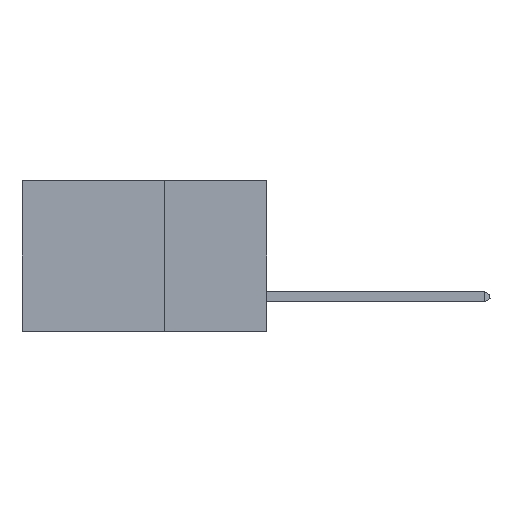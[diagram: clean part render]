
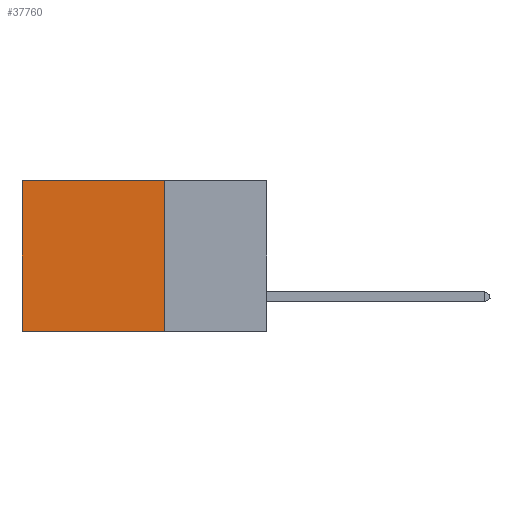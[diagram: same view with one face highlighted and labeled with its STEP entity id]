
A CAD part, left-side view. The second image highlights one B-rep face of the part: STEP entity #37760.
In plain terms, the highlighted planar face has unit normal (-1, 0, 0).
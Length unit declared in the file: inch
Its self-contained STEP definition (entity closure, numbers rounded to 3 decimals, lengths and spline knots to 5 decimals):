
#5475 = VECTOR ( 'NONE', #35200, 39.37008 ) ;
#6870 = VECTOR ( 'NONE', #21908, 39.37008 ) ;
#8122 = CARTESIAN_POINT ( 'NONE',  ( 0.2875, 0.25, 0. ) ) ;
#8589 = FACE_OUTER_BOUND ( 'NONE', #17718, .T. ) ;
#9537 = CARTESIAN_POINT ( 'NONE',  ( 0.2875, 0.25, -0.37 ) ) ;
#10357 = ORIENTED_EDGE ( 'NONE', *, *, #39646, .F. ) ;
#11465 = DIRECTION ( 'NONE',  ( 1., 0., 0. ) ) ;
#13962 = CARTESIAN_POINT ( 'NONE',  ( 0.2875, 0.6, 0. ) ) ;
#14576 = LINE ( 'NONE', #37677, #35954 ) ;
#15510 = EDGE_CURVE ( 'NONE', #18919, #43101, #44362, .T. ) ;
#15926 = CARTESIAN_POINT ( 'NONE',  ( 0.2875, 0.25, 0. ) ) ;
#16821 = LINE ( 'NONE', #13962, #6870 ) ;
#17718 = EDGE_LOOP ( 'NONE', ( #42043, #27806, #10357, #18698 ) ) ;
#17753 = VECTOR ( 'NONE', #43598, 39.37008 ) ;
#18698 = ORIENTED_EDGE ( 'NONE', *, *, #42500, .T. ) ;
#18919 = VERTEX_POINT ( 'NONE', #36435 ) ;
#21020 = EDGE_CURVE ( 'NONE', #38689, #43101, #16821, .T. ) ;
#21908 = DIRECTION ( 'NONE',  ( 0., 0., -1. ) ) ;
#25584 = LINE ( 'NONE', #15926, #5475 ) ;
#27806 = ORIENTED_EDGE ( 'NONE', *, *, #15510, .F. ) ;
#33387 = AXIS2_PLACEMENT_3D ( 'NONE', #8122, #11465, #42192 ) ;
#34142 = PLANE ( 'NONE',  #33387 ) ;
#35200 = DIRECTION ( 'NONE',  ( 0., 0., -1. ) ) ;
#35954 = VECTOR ( 'NONE', #45990, 39.37008 ) ;
#36435 = CARTESIAN_POINT ( 'NONE',  ( 0.2875, 0.25, -0.37 ) ) ;
#37048 = CARTESIAN_POINT ( 'NONE',  ( 0.2875, 0.6, 0. ) ) ;
#37677 = CARTESIAN_POINT ( 'NONE',  ( 0.2875, 0.25, 0. ) ) ;
#37760 = ADVANCED_FACE ( 'NONE', ( #8589 ), #34142, .F. ) ;
#38689 = VERTEX_POINT ( 'NONE', #37048 ) ;
#39646 = EDGE_CURVE ( 'NONE', #40499, #18919, #25584, .T. ) ;
#40436 = CARTESIAN_POINT ( 'NONE',  ( 0.2875, 0.6, -0.37 ) ) ;
#40499 = VERTEX_POINT ( 'NONE', #48067 ) ;
#42043 = ORIENTED_EDGE ( 'NONE', *, *, #21020, .T. ) ;
#42192 = DIRECTION ( 'NONE',  ( 0., 0., -1. ) ) ;
#42500 = EDGE_CURVE ( 'NONE', #40499, #38689, #14576, .T. ) ;
#43101 = VERTEX_POINT ( 'NONE', #40436 ) ;
#43598 = DIRECTION ( 'NONE',  ( 0., 1., 0. ) ) ;
#44362 = LINE ( 'NONE', #9537, #17753 ) ;
#45990 = DIRECTION ( 'NONE',  ( 0., 1., 0. ) ) ;
#48067 = CARTESIAN_POINT ( 'NONE',  ( 0.2875, 0.25, 0. ) ) ;
